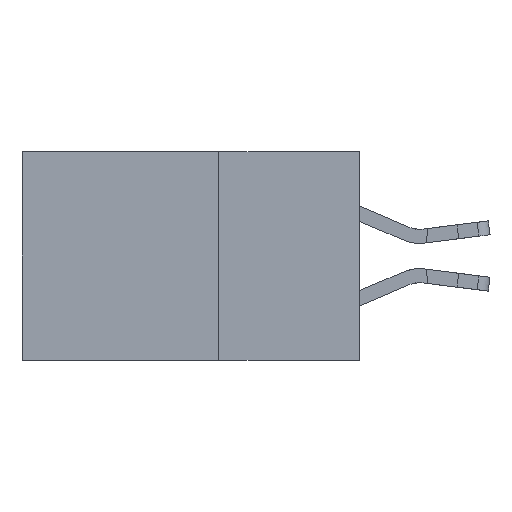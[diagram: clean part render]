
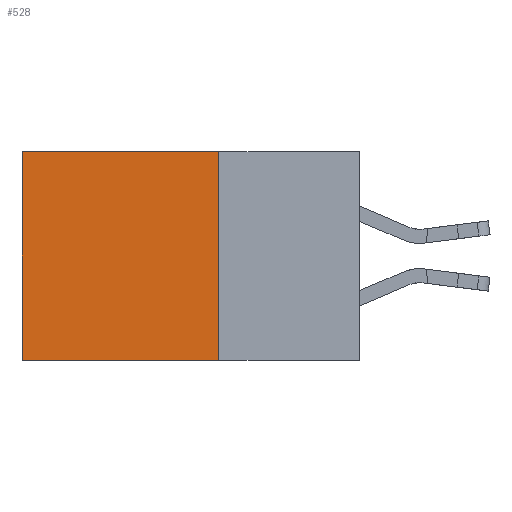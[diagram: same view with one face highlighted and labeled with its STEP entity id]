
A CAD part, left-side view. The second image highlights one B-rep face of the part: STEP entity #528.
In plain terms, the highlighted planar face has unit normal (-1, 0, 0).
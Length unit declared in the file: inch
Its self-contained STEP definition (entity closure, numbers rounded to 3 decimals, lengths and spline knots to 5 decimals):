
#417 = CARTESIAN_POINT ( 'NONE',  ( 0.2875, 0.25, 0. ) ) ;
#528 = ADVANCED_FACE ( 'NONE', ( #19715 ), #7033, .F. ) ;
#582 = VECTOR ( 'NONE', #9767, 39.37008 ) ;
#1222 = AXIS2_PLACEMENT_3D ( 'NONE', #2642, #8756, #7127 ) ;
#1478 = VERTEX_POINT ( 'NONE', #2923 ) ;
#1763 = VECTOR ( 'NONE', #5226, 39.37008 ) ;
#2407 = CARTESIAN_POINT ( 'NONE',  ( 0.2875, 0.6, 0. ) ) ;
#2642 = CARTESIAN_POINT ( 'NONE',  ( 0.2875, 0.25, 0. ) ) ;
#2923 = CARTESIAN_POINT ( 'NONE',  ( 0.2875, 0.25, 0. ) ) ;
#5226 = DIRECTION ( 'NONE',  ( 0., 0., -1. ) ) ;
#6059 = CARTESIAN_POINT ( 'NONE',  ( 0.2875, 0.25, -0.37 ) ) ;
#6988 = LINE ( 'NONE', #2407, #16075 ) ;
#7019 = LINE ( 'NONE', #417, #582 ) ;
#7033 = PLANE ( 'NONE',  #1222 ) ;
#7067 = CARTESIAN_POINT ( 'NONE',  ( 0.2875, 0.6, 0. ) ) ;
#7127 = DIRECTION ( 'NONE',  ( 0., 0., -1. ) ) ;
#7801 = VECTOR ( 'NONE', #9313, 39.37008 ) ;
#7886 = LINE ( 'NONE', #6059, #7801 ) ;
#8191 = EDGE_LOOP ( 'NONE', ( #15816, #11502, #19527, #17035 ) ) ;
#8512 = DIRECTION ( 'NONE',  ( 0., 0., -1. ) ) ;
#8746 = EDGE_CURVE ( 'NONE', #1478, #14525, #11330, .T. ) ;
#8756 = DIRECTION ( 'NONE',  ( 1., 0., 0. ) ) ;
#9313 = DIRECTION ( 'NONE',  ( 0., 1., 0. ) ) ;
#9767 = DIRECTION ( 'NONE',  ( 0., 1., 0. ) ) ;
#11330 = LINE ( 'NONE', #17602, #1763 ) ;
#11502 = ORIENTED_EDGE ( 'NONE', *, *, #17212, .F. ) ;
#11709 = EDGE_CURVE ( 'NONE', #15833, #19503, #6988, .T. ) ;
#12100 = CARTESIAN_POINT ( 'NONE',  ( 0.2875, 0.25, -0.37 ) ) ;
#12793 = CARTESIAN_POINT ( 'NONE',  ( 0.2875, 0.6, -0.37 ) ) ;
#14525 = VERTEX_POINT ( 'NONE', #12100 ) ;
#14741 = EDGE_CURVE ( 'NONE', #1478, #15833, #7019, .T. ) ;
#15816 = ORIENTED_EDGE ( 'NONE', *, *, #11709, .T. ) ;
#15833 = VERTEX_POINT ( 'NONE', #7067 ) ;
#16075 = VECTOR ( 'NONE', #8512, 39.37008 ) ;
#17035 = ORIENTED_EDGE ( 'NONE', *, *, #14741, .T. ) ;
#17212 = EDGE_CURVE ( 'NONE', #14525, #19503, #7886, .T. ) ;
#17602 = CARTESIAN_POINT ( 'NONE',  ( 0.2875, 0.25, 0. ) ) ;
#19503 = VERTEX_POINT ( 'NONE', #12793 ) ;
#19527 = ORIENTED_EDGE ( 'NONE', *, *, #8746, .F. ) ;
#19715 = FACE_OUTER_BOUND ( 'NONE', #8191, .T. ) ;
